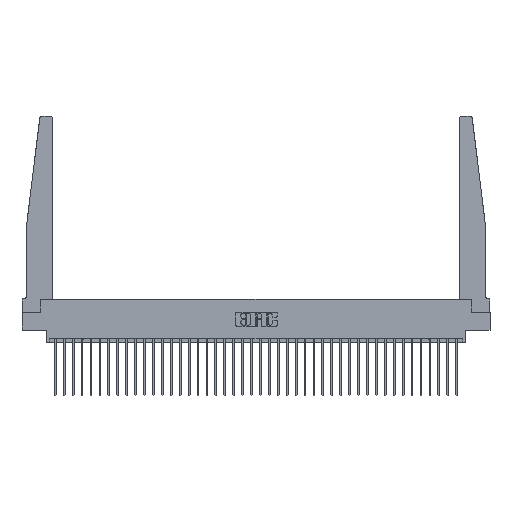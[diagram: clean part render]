
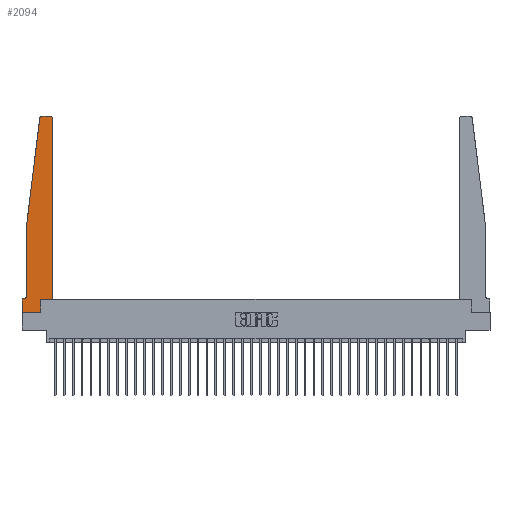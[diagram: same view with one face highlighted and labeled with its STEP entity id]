
A CAD part, top view. The second image highlights one B-rep face of the part: STEP entity #2094.
In plain terms, the highlighted planar face has unit normal (0, 0, 1).
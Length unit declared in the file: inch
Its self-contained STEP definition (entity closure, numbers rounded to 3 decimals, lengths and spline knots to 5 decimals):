
#509 = CARTESIAN_POINT ( 'NONE',  ( 0.015, 0.2375, 0.37 ) ) ;
#643 = EDGE_CURVE ( 'NONE', #28695, #28204, #11828, .T. ) ;
#750 = VECTOR ( 'NONE', #18697, 39.37008 ) ;
#1908 = EDGE_CURVE ( 'NONE', #8615, #18388, #24261, .T. ) ;
#2094 = ADVANCED_FACE ( 'NONE', ( #3437 ), #23144, .T. ) ;
#2834 = EDGE_CURVE ( 'NONE', #31167, #17325, #24333, .T. ) ;
#2859 = ORIENTED_EDGE ( 'NONE', *, *, #17747, .T. ) ;
#2955 = LINE ( 'NONE', #5287, #9252 ) ;
#3219 = DIRECTION ( 'NONE',  ( -1., 0., 0. ) ) ;
#3437 = FACE_OUTER_BOUND ( 'NONE', #10811, .T. ) ;
#4543 = CARTESIAN_POINT ( 'NONE',  ( 0., 0.1875, 0.37 ) ) ;
#5016 = VECTOR ( 'NONE', #23844, 39.37008 ) ;
#5287 = CARTESIAN_POINT ( 'NONE',  ( 0.2605, 0.18, 0.37 ) ) ;
#5356 = CARTESIAN_POINT ( 'NONE',  ( 0., 0., 0.37 ) ) ;
#5851 = ORIENTED_EDGE ( 'NONE', *, *, #21551, .T. ) ;
#6437 = VERTEX_POINT ( 'NONE', #16246 ) ;
#6587 = DIRECTION ( 'NONE',  ( -0.122, -0.992, 0. ) ) ;
#6692 = ORIENTED_EDGE ( 'NONE', *, *, #1908, .T. ) ;
#7061 = CARTESIAN_POINT ( 'NONE',  ( 0.425, 2.72, 0.37 ) ) ;
#7089 = VERTEX_POINT ( 'NONE', #16317 ) ;
#7148 = DIRECTION ( 'NONE',  ( 0., 1., 0. ) ) ;
#7232 = DIRECTION ( 'NONE',  ( 0., 0., 1. ) ) ;
#7614 = VERTEX_POINT ( 'NONE', #10321 ) ;
#8124 = CARTESIAN_POINT ( 'NONE',  ( 0.065, 0.2375, 0.37 ) ) ;
#8473 = AXIS2_PLACEMENT_3D ( 'NONE', #509, #19175, #3219 ) ;
#8509 = CARTESIAN_POINT ( 'NONE',  ( 0.395, 2.75, 0.37 ) ) ;
#8615 = VERTEX_POINT ( 'NONE', #19326 ) ;
#9061 = ORIENTED_EDGE ( 'NONE', *, *, #2834, .T. ) ;
#9252 = VECTOR ( 'NONE', #26577, 39.37008 ) ;
#9637 = LINE ( 'NONE', #25961, #22936 ) ;
#10321 = CARTESIAN_POINT ( 'NONE',  ( 0.2605, 0., 0.37 ) ) ;
#10811 = EDGE_LOOP ( 'NONE', ( #26497, #12589, #18505, #28000, #23163, #5851, #28536, #2859, #26911, #6692, #30247, #9061 ) ) ;
#11280 = EDGE_CURVE ( 'NONE', #32060, #23052, #27724, .T. ) ;
#11828 = CIRCLE ( 'NONE', #13431, 0.03 ) ;
#12589 = ORIENTED_EDGE ( 'NONE', *, *, #643, .T. ) ;
#13023 = AXIS2_PLACEMENT_3D ( 'NONE', #13109, #31632, #15785 ) ;
#13109 = CARTESIAN_POINT ( 'NONE',  ( 0.395, 2.72, 0.37 ) ) ;
#13431 = AXIS2_PLACEMENT_3D ( 'NONE', #14525, #33031, #17178 ) ;
#14525 = CARTESIAN_POINT ( 'NONE',  ( 0.27653, 2.72, 0.37 ) ) ;
#14575 = EDGE_CURVE ( 'NONE', #29588, #32060, #34126, .T. ) ;
#15168 = EDGE_CURVE ( 'NONE', #17325, #28695, #9637, .T. ) ;
#15665 = DIRECTION ( 'NONE',  ( 0., -1., 0. ) ) ;
#15785 = DIRECTION ( 'NONE',  ( 1., 0., 0. ) ) ;
#16246 = CARTESIAN_POINT ( 'NONE',  ( 0., 0., 0.37 ) ) ;
#16317 = CARTESIAN_POINT ( 'NONE',  ( 0., 0.1875, 0.37 ) ) ;
#16564 = EDGE_CURVE ( 'NONE', #7614, #8615, #2955, .T. ) ;
#16709 = CARTESIAN_POINT ( 'NONE',  ( 0.015, 0.1875, 0.37 ) ) ;
#17178 = DIRECTION ( 'NONE',  ( 1., 0., 0. ) ) ;
#17193 = EDGE_CURVE ( 'NONE', #7089, #6437, #33245, .T. ) ;
#17325 = VERTEX_POINT ( 'NONE', #8509 ) ;
#17747 = EDGE_CURVE ( 'NONE', #6437, #7614, #29093, .T. ) ;
#17900 = AXIS2_PLACEMENT_3D ( 'NONE', #4543, #7232, #25820 ) ;
#18388 = VERTEX_POINT ( 'NONE', #29223 ) ;
#18505 = ORIENTED_EDGE ( 'NONE', *, *, #32299, .T. ) ;
#18697 = DIRECTION ( 'NONE',  ( 1., 0., 0. ) ) ;
#19175 = DIRECTION ( 'NONE',  ( 0., 0., -1. ) ) ;
#19326 = CARTESIAN_POINT ( 'NONE',  ( 0.2605, 0.18, 0.37 ) ) ;
#19832 = CARTESIAN_POINT ( 'NONE',  ( 0.065, 1.25, 0.37 ) ) ;
#20361 = EDGE_CURVE ( 'NONE', #18388, #31167, #26086, .T. ) ;
#20747 = CARTESIAN_POINT ( 'NONE',  ( 0.065, 1.25, 0.37 ) ) ;
#21551 = EDGE_CURVE ( 'NONE', #23052, #7089, #33423, .T. ) ;
#22444 = CARTESIAN_POINT ( 'NONE',  ( 0.425, 0.18, 0.37 ) ) ;
#22936 = VECTOR ( 'NONE', #23497, 39.37008 ) ;
#23052 = VERTEX_POINT ( 'NONE', #16709 ) ;
#23061 = CARTESIAN_POINT ( 'NONE',  ( 0.425, 0.18, 0.37 ) ) ;
#23144 = PLANE ( 'NONE',  #17900 ) ;
#23163 = ORIENTED_EDGE ( 'NONE', *, *, #11280, .T. ) ;
#23422 = VECTOR ( 'NONE', #25124, 39.37008 ) ;
#23497 = DIRECTION ( 'NONE',  ( -1., 0., 0. ) ) ;
#23538 = CARTESIAN_POINT ( 'NONE',  ( 0.065, 1.25, 0.37 ) ) ;
#23844 = DIRECTION ( 'NONE',  ( 0., -1., 0. ) ) ;
#24261 = LINE ( 'NONE', #22444, #23422 ) ;
#24333 = CIRCLE ( 'NONE', #13023, 0.03 ) ;
#24383 = VECTOR ( 'NONE', #6587, 39.37008 ) ;
#24817 = CARTESIAN_POINT ( 'NONE',  ( 0.24675, 2.72367, 0.37 ) ) ;
#24963 = DIRECTION ( 'NONE',  ( -1., 0., 0. ) ) ;
#25124 = DIRECTION ( 'NONE',  ( 1., 0., 0. ) ) ;
#25685 = CARTESIAN_POINT ( 'NONE',  ( 0.27653, 2.75, 0.37 ) ) ;
#25820 = DIRECTION ( 'NONE',  ( 1., 0., 0. ) ) ;
#25961 = CARTESIAN_POINT ( 'NONE',  ( 0.25, 2.75, 0.37 ) ) ;
#26076 = LINE ( 'NONE', #19832, #24383 ) ;
#26086 = LINE ( 'NONE', #23061, #33088 ) ;
#26497 = ORIENTED_EDGE ( 'NONE', *, *, #15168, .T. ) ;
#26577 = DIRECTION ( 'NONE',  ( 0., 1., 0. ) ) ;
#26911 = ORIENTED_EDGE ( 'NONE', *, *, #16564, .T. ) ;
#27127 = VECTOR ( 'NONE', #15665, 39.37008 ) ;
#27724 = CIRCLE ( 'NONE', #8473, 0.05 ) ;
#28000 = ORIENTED_EDGE ( 'NONE', *, *, #14575, .T. ) ;
#28204 = VERTEX_POINT ( 'NONE', #24817 ) ;
#28536 = ORIENTED_EDGE ( 'NONE', *, *, #17193, .T. ) ;
#28695 = VERTEX_POINT ( 'NONE', #25685 ) ;
#29093 = LINE ( 'NONE', #31884, #750 ) ;
#29223 = CARTESIAN_POINT ( 'NONE',  ( 0.425, 0.18, 0.37 ) ) ;
#29588 = VERTEX_POINT ( 'NONE', #20747 ) ;
#30164 = CARTESIAN_POINT ( 'NONE',  ( 0.065, 0.1875, 0.37 ) ) ;
#30247 = ORIENTED_EDGE ( 'NONE', *, *, #20361, .T. ) ;
#31167 = VERTEX_POINT ( 'NONE', #7061 ) ;
#31632 = DIRECTION ( 'NONE',  ( 0., 0., 1. ) ) ;
#31754 = VECTOR ( 'NONE', #24963, 39.37008 ) ;
#31884 = CARTESIAN_POINT ( 'NONE',  ( 0., 0., 0.37 ) ) ;
#32060 = VERTEX_POINT ( 'NONE', #8124 ) ;
#32299 = EDGE_CURVE ( 'NONE', #28204, #29588, #26076, .T. ) ;
#33031 = DIRECTION ( 'NONE',  ( 0., 0., 1. ) ) ;
#33088 = VECTOR ( 'NONE', #7148, 39.37008 ) ;
#33245 = LINE ( 'NONE', #5356, #5016 ) ;
#33423 = LINE ( 'NONE', #30164, #31754 ) ;
#34126 = LINE ( 'NONE', #23538, #27127 ) ;
